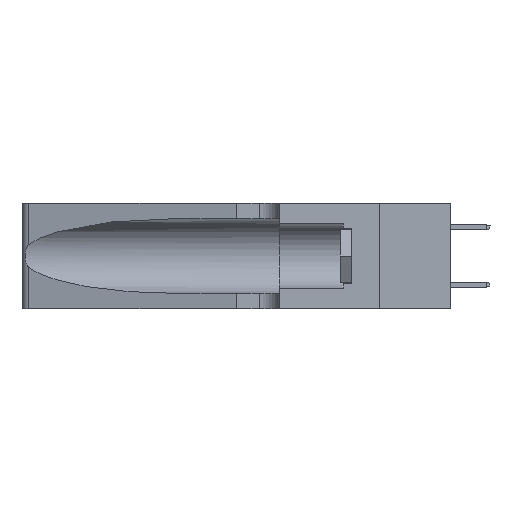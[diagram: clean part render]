
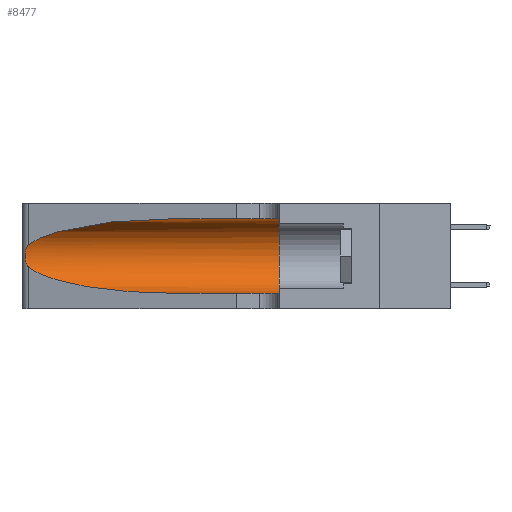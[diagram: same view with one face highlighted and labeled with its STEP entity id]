
A CAD part, left-side view. The second image highlights one B-rep face of the part: STEP entity #8477.
In plain terms, the highlighted cylindrical face has radius 3.308 mm (diameter 6.617 mm), a partial arc.
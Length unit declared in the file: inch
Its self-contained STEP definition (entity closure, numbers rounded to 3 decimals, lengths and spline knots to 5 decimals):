
#117 = VECTOR ( 'NONE', #8817, 39.37008 ) ;
#509 = DIRECTION ( 'NONE',  ( 0., 0., -1. ) ) ;
#1196 = VERTEX_POINT ( 'NONE', #16310 ) ;
#1361 = CARTESIAN_POINT ( 'NONE',  ( 0.25639, 1.23184, 0.21858 ) ) ;
#1721 = CARTESIAN_POINT ( 'NONE',  ( 0.25639, 1.23186, 0.15144 ) ) ;
#1905 = CARTESIAN_POINT ( 'NONE',  ( 0.25487, 1.22718, 0.22369 ) ) ;
#2271 = CARTESIAN_POINT ( 'NONE',  ( 0.1305, 0.35, 0.31525 ) ) ;
#2372 = EDGE_LOOP ( 'NONE', ( #10274, #8593, #16241, #16598, #19022, #19699 ) ) ;
#2583 = VERTEX_POINT ( 'NONE', #1905 ) ;
#3519 = CARTESIAN_POINT ( 'NONE',  ( 0.25487, 1.22718, 0.22369 ) ) ;
#3540 = CARTESIAN_POINT ( 'NONE',  ( 0.1305, 1.61858, 0.31525 ) ) ;
#3817 = VERTEX_POINT ( 'NONE', #2271 ) ;
#5099 = DIRECTION ( 'NONE',  ( 0., 1., 0. ) ) ;
#5375 = AXIS2_PLACEMENT_3D ( 'NONE', #18724, #11600, #509 ) ;
#6257 = VERTEX_POINT ( 'NONE', #9158 ) ;
#6854 = CARTESIAN_POINT ( 'NONE',  ( 0.25487, 1.22718, 0.14631 ) ) ;
#6980 = CARTESIAN_POINT ( 'NONE',  ( 0.25854, 1.2359, 0.20912 ) ) ;
#7202 = CARTESIAN_POINT ( 'NONE',  ( 0.25555, 1.22993, 0.14849 ) ) ;
#8332 = CARTESIAN_POINT ( 'NONE',  ( 0.25487, 1.22718, 0.22369 ) ) ;
#8477 = ADVANCED_FACE ( 'NONE', ( #20267 ), #19074, .F. ) ;
#8593 = ORIENTED_EDGE ( 'NONE', *, *, #18697, .T. ) ;
#8640 = CARTESIAN_POINT ( 'NONE',  ( 0.26075, 1.23896, 0.19203 ) ) ;
#8683 =( BOUNDED_CURVE ( )  B_SPLINE_CURVE ( 3, ( #9145, #10691, #19725, #19842 ),
 .UNSPECIFIED., .F., .F. ) 
 B_SPLINE_CURVE_WITH_KNOTS ( ( 4, 4 ),
 ( 3.44316, 4.71239 ),
 .UNSPECIFIED. ) 
 CURVE ( )  GEOMETRIC_REPRESENTATION_ITEM ( )  RATIONAL_B_SPLINE_CURVE ( ( 1., 0.87, 0.87, 1. ) ) 
 REPRESENTATION_ITEM ( '' )  );
#8817 = DIRECTION ( 'NONE',  ( 0., -1., 0. ) ) ;
#8978 = VERTEX_POINT ( 'NONE', #21899 ) ;
#9017 = CARTESIAN_POINT ( 'NONE',  ( 0.1305, 0.35, 0.185 ) ) ;
#9132 = EDGE_CURVE ( 'NONE', #6257, #3817, #19482, .T. ) ;
#9145 = CARTESIAN_POINT ( 'NONE',  ( 0.25487, 1.22718, 0.14631 ) ) ;
#9158 = CARTESIAN_POINT ( 'NONE',  ( 0.1305, 0.72297, 0.31525 ) ) ;
#9186 = EDGE_CURVE ( 'NONE', #3817, #12601, #11867, .T. ) ;
#10274 = ORIENTED_EDGE ( 'NONE', *, *, #22736, .T. ) ;
#10661 = CARTESIAN_POINT ( 'NONE',  ( 0.25787, 1.23484, 0.2124 ) ) ;
#10691 = CARTESIAN_POINT ( 'NONE',  ( 0.2373, 1.15595, 0.08982 ) ) ;
#10718 = LINE ( 'NONE', #15836, #117 ) ;
#10889 = EDGE_CURVE ( 'NONE', #1196, #12601, #10718, .T. ) ;
#11600 = DIRECTION ( 'NONE',  ( 0., -1., 0. ) ) ;
#11867 = CIRCLE ( 'NONE', #17546, 0.13025 ) ;
#12148 = CARTESIAN_POINT ( 'NONE',  ( 0.2373, 1.15595, 0.28018 ) ) ;
#12601 = VERTEX_POINT ( 'NONE', #19267 ) ;
#13805 = CARTESIAN_POINT ( 'NONE',  ( 0.1305, 0.72297, 0.31525 ) ) ;
#15836 = CARTESIAN_POINT ( 'NONE',  ( 0.1305, 1.61858, 0.05475 ) ) ;
#15890 = CARTESIAN_POINT ( 'NONE',  ( 0.26075, 1.23896, 0.178 ) ) ;
#16241 = ORIENTED_EDGE ( 'NONE', *, *, #18181, .T. ) ;
#16251 = DIRECTION ( 'NONE',  ( 0., -1., 0. ) ) ;
#16310 = CARTESIAN_POINT ( 'NONE',  ( 0.1305, 0.72297, 0.05475 ) ) ;
#16598 = ORIENTED_EDGE ( 'NONE', *, *, #10889, .T. ) ;
#17546 = AXIS2_PLACEMENT_3D ( 'NONE', #9017, #5099, #17929 ) ;
#17929 = DIRECTION ( 'NONE',  ( 0., 0., 1. ) ) ;
#18027 = CARTESIAN_POINT ( 'NONE',  ( 0.26017, 1.23833, 0.17102 ) ) ;
#18181 = EDGE_CURVE ( 'NONE', #8978, #1196, #8683, .T. ) ;
#18400 = B_SPLINE_CURVE_WITH_KNOTS ( 'NONE', 3,
 ( #3519, #23253, #1361, #10661, #6980, #19693, #8640, #15890, #18027, #23138, #21351, #1721, #7202, #6854 ),
 .UNSPECIFIED., .F., .F.,
 ( 4, 2, 2, 2, 2, 2, 4 ),
 ( 0., 0.00027, 0.00053, 0.00107, 0.0016, 0.00187, 0.00214 ),
 .UNSPECIFIED. ) ;
#18697 = EDGE_CURVE ( 'NONE', #2583, #8978, #18400, .T. ) ;
#18724 = CARTESIAN_POINT ( 'NONE',  ( 0.1305, 1.61858, 0.185 ) ) ;
#19022 = ORIENTED_EDGE ( 'NONE', *, *, #9186, .F. ) ;
#19074 = CYLINDRICAL_SURFACE ( 'NONE', #5375, 0.13025 ) ;
#19267 = CARTESIAN_POINT ( 'NONE',  ( 0.1305, 0.35, 0.05475 ) ) ;
#19482 = LINE ( 'NONE', #3540, #23247 ) ;
#19693 = CARTESIAN_POINT ( 'NONE',  ( 0.26018, 1.23835, 0.19895 ) ) ;
#19699 = ORIENTED_EDGE ( 'NONE', *, *, #9132, .F. ) ;
#19725 = CARTESIAN_POINT ( 'NONE',  ( 0.18966, 0.96281, 0.05475 ) ) ;
#19842 = CARTESIAN_POINT ( 'NONE',  ( 0.1305, 0.72297, 0.05475 ) ) ;
#20267 = FACE_OUTER_BOUND ( 'NONE', #2372, .T. ) ;
#20833 =( BOUNDED_CURVE ( )  B_SPLINE_CURVE ( 3, ( #13805, #22715, #12148, #8332 ),
 .UNSPECIFIED., .F., .F. ) 
 B_SPLINE_CURVE_WITH_KNOTS ( ( 4, 4 ),
 ( 1.5708, 2.84003 ),
 .UNSPECIFIED. ) 
 CURVE ( )  GEOMETRIC_REPRESENTATION_ITEM ( )  RATIONAL_B_SPLINE_CURVE ( ( 1., 0.87, 0.87, 1. ) ) 
 REPRESENTATION_ITEM ( '' )  );
#21351 = CARTESIAN_POINT ( 'NONE',  ( 0.25789, 1.23486, 0.15765 ) ) ;
#21899 = CARTESIAN_POINT ( 'NONE',  ( 0.25487, 1.22718, 0.14631 ) ) ;
#22715 = CARTESIAN_POINT ( 'NONE',  ( 0.18966, 0.96281, 0.31525 ) ) ;
#22736 = EDGE_CURVE ( 'NONE', #6257, #2583, #20833, .T. ) ;
#23138 = CARTESIAN_POINT ( 'NONE',  ( 0.25856, 1.23593, 0.16098 ) ) ;
#23247 = VECTOR ( 'NONE', #16251, 39.37008 ) ;
#23253 = CARTESIAN_POINT ( 'NONE',  ( 0.25555, 1.22994, 0.2215 ) ) ;
